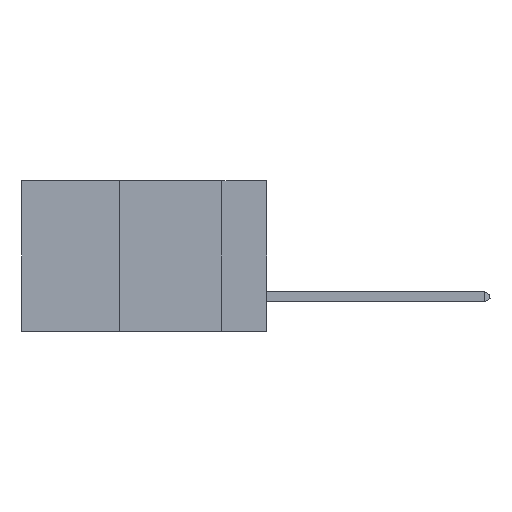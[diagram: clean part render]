
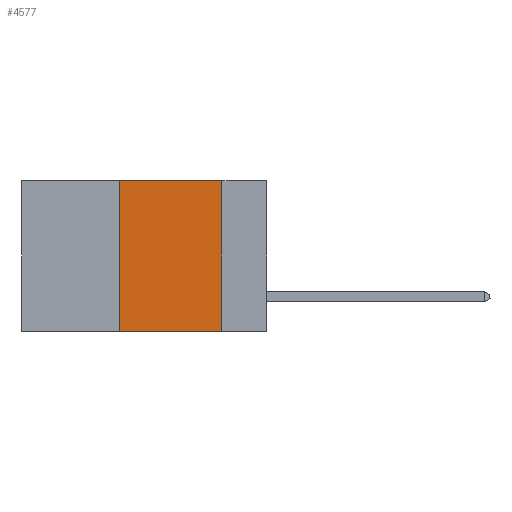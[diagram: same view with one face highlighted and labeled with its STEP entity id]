
A CAD part, left-side view. The second image highlights one B-rep face of the part: STEP entity #4577.
In plain terms, the highlighted planar face has unit normal (-1, 0, 0).
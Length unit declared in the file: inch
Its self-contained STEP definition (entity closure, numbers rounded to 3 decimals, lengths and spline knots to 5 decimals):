
#1374 = VERTEX_POINT ( 'NONE', #26371 ) ;
#1401 = LINE ( 'NONE', #27506, #28154 ) ;
#1662 = DIRECTION ( 'NONE',  ( 0., 0., -1. ) ) ;
#1867 = DIRECTION ( 'NONE',  ( 0., -1., 0. ) ) ;
#3808 = ORIENTED_EDGE ( 'NONE', *, *, #16469, .F. ) ;
#4042 = ORIENTED_EDGE ( 'NONE', *, *, #29462, .F. ) ;
#4577 = ADVANCED_FACE ( 'NONE', ( #23085 ), #33205, .F. ) ;
#4625 = CARTESIAN_POINT ( 'NONE',  ( 0., 0.11, 0. ) ) ;
#4817 = DIRECTION ( 'NONE',  ( 0., 0., -1. ) ) ;
#5142 = CARTESIAN_POINT ( 'NONE',  ( 0., 0.11, -0.37 ) ) ;
#7324 = DIRECTION ( 'NONE',  ( 0., -1., 0. ) ) ;
#8014 = VECTOR ( 'NONE', #7324, 39.37008 ) ;
#9121 = CARTESIAN_POINT ( 'NONE',  ( 0., 0.36, 0. ) ) ;
#9506 = VERTEX_POINT ( 'NONE', #26754 ) ;
#9596 = ORIENTED_EDGE ( 'NONE', *, *, #27031, .F. ) ;
#13791 = EDGE_CURVE ( 'NONE', #1374, #26529, #28725, .T. ) ;
#15220 = CARTESIAN_POINT ( 'NONE',  ( 0., 0.6, 0. ) ) ;
#16469 = EDGE_CURVE ( 'NONE', #16719, #26529, #1401, .T. ) ;
#16719 = VERTEX_POINT ( 'NONE', #4625 ) ;
#18857 = EDGE_LOOP ( 'NONE', ( #3808, #9596, #4042, #19204 ) ) ;
#19204 = ORIENTED_EDGE ( 'NONE', *, *, #13791, .T. ) ;
#19439 = VECTOR ( 'NONE', #1867, 39.37008 ) ;
#19788 = AXIS2_PLACEMENT_3D ( 'NONE', #15220, #33302, #4817 ) ;
#20628 = LINE ( 'NONE', #22530, #19439 ) ;
#22530 = CARTESIAN_POINT ( 'NONE',  ( 0., 0.6, 0. ) ) ;
#23085 = FACE_OUTER_BOUND ( 'NONE', #18857, .T. ) ;
#24342 = VECTOR ( 'NONE', #24561, 39.37008 ) ;
#24561 = DIRECTION ( 'NONE',  ( 0., 0., 1. ) ) ;
#26371 = CARTESIAN_POINT ( 'NONE',  ( 0., 0.36, -0.37 ) ) ;
#26529 = VERTEX_POINT ( 'NONE', #5142 ) ;
#26754 = CARTESIAN_POINT ( 'NONE',  ( 0., 0.36, 0. ) ) ;
#27031 = EDGE_CURVE ( 'NONE', #9506, #16719, #20628, .T. ) ;
#27506 = CARTESIAN_POINT ( 'NONE',  ( 0., 0.11, 0. ) ) ;
#28154 = VECTOR ( 'NONE', #1662, 39.37008 ) ;
#28202 = CARTESIAN_POINT ( 'NONE',  ( 0., 0.6, -0.37 ) ) ;
#28725 = LINE ( 'NONE', #28202, #8014 ) ;
#29462 = EDGE_CURVE ( 'NONE', #1374, #9506, #33246, .T. ) ;
#33205 = PLANE ( 'NONE',  #19788 ) ;
#33246 = LINE ( 'NONE', #9121, #24342 ) ;
#33302 = DIRECTION ( 'NONE',  ( 1., 0., 0. ) ) ;
